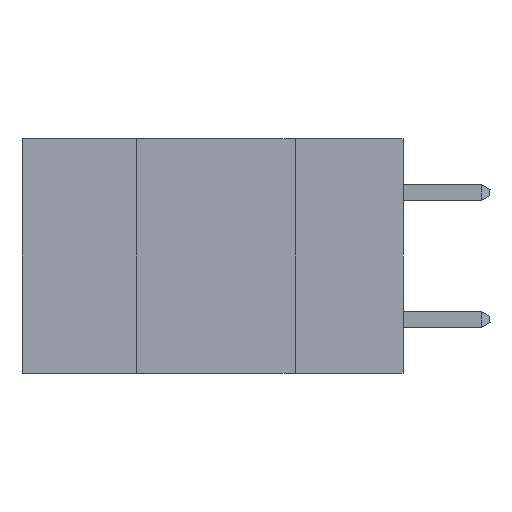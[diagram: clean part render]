
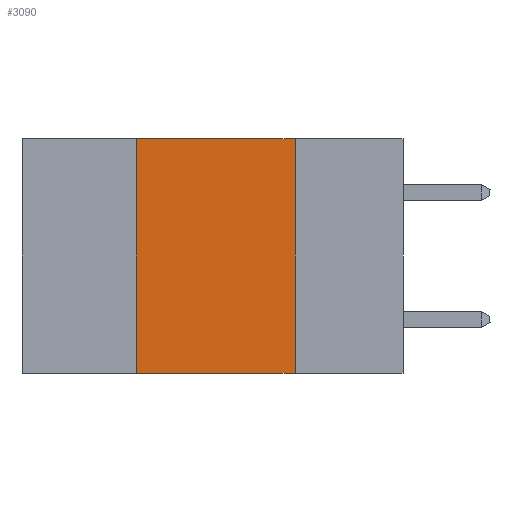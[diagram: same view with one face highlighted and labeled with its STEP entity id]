
A CAD part, left-side view. The second image highlights one B-rep face of the part: STEP entity #3090.
In plain terms, the highlighted planar face has unit normal (-1, 0, 0).
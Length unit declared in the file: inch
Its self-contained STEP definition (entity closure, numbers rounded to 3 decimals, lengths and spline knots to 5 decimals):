
#54 = EDGE_CURVE ( 'NONE', #2871, #9619, #1318, .T. ) ;
#426 = DIRECTION ( 'NONE',  ( 1., 0., 0. ) ) ;
#457 = AXIS2_PLACEMENT_3D ( 'NONE', #13632, #426, #7081 ) ;
#460 = CARTESIAN_POINT ( 'NONE',  ( 0., 0.42, 0. ) ) ;
#549 = EDGE_CURVE ( 'NONE', #13292, #9970, #6800, .T. ) ;
#629 = CARTESIAN_POINT ( 'NONE',  ( 0., 0.42, 0. ) ) ;
#1159 = VECTOR ( 'NONE', #8277, 39.37008 ) ;
#1318 = LINE ( 'NONE', #7548, #12963 ) ;
#2871 = VERTEX_POINT ( 'NONE', #11934 ) ;
#3051 = LINE ( 'NONE', #3916, #1159 ) ;
#3090 = ADVANCED_FACE ( 'NONE', ( #12786 ), #10303, .F. ) ;
#3916 = CARTESIAN_POINT ( 'NONE',  ( 0., 0.17, 0. ) ) ;
#4755 = CARTESIAN_POINT ( 'NONE',  ( 0., 0.17, -0.37 ) ) ;
#5334 = EDGE_CURVE ( 'NONE', #2871, #13292, #7919, .T. ) ;
#5450 = ORIENTED_EDGE ( 'NONE', *, *, #549, .F. ) ;
#5946 = DIRECTION ( 'NONE',  ( 0., 0., 1. ) ) ;
#6522 = CARTESIAN_POINT ( 'NONE',  ( 0., 0.17, 0. ) ) ;
#6800 = LINE ( 'NONE', #8638, #11696 ) ;
#7081 = DIRECTION ( 'NONE',  ( 0., 0., -1. ) ) ;
#7548 = CARTESIAN_POINT ( 'NONE',  ( 0., 0.6, -0.37 ) ) ;
#7919 = LINE ( 'NONE', #629, #8254 ) ;
#8254 = VECTOR ( 'NONE', #5946, 39.37008 ) ;
#8277 = DIRECTION ( 'NONE',  ( 0., 0., -1. ) ) ;
#8453 = DIRECTION ( 'NONE',  ( 0., -1., 0. ) ) ;
#8638 = CARTESIAN_POINT ( 'NONE',  ( 0., 0.6, 0. ) ) ;
#9619 = VERTEX_POINT ( 'NONE', #4755 ) ;
#9970 = VERTEX_POINT ( 'NONE', #6522 ) ;
#10150 = EDGE_LOOP ( 'NONE', ( #13589, #5450, #11818, #12194 ) ) ;
#10303 = PLANE ( 'NONE',  #457 ) ;
#10901 = DIRECTION ( 'NONE',  ( 0., -1., 0. ) ) ;
#11696 = VECTOR ( 'NONE', #8453, 39.37008 ) ;
#11818 = ORIENTED_EDGE ( 'NONE', *, *, #5334, .F. ) ;
#11934 = CARTESIAN_POINT ( 'NONE',  ( 0., 0.42, -0.37 ) ) ;
#12194 = ORIENTED_EDGE ( 'NONE', *, *, #54, .T. ) ;
#12786 = FACE_OUTER_BOUND ( 'NONE', #10150, .T. ) ;
#12963 = VECTOR ( 'NONE', #10901, 39.37008 ) ;
#13292 = VERTEX_POINT ( 'NONE', #460 ) ;
#13589 = ORIENTED_EDGE ( 'NONE', *, *, #14063, .F. ) ;
#13632 = CARTESIAN_POINT ( 'NONE',  ( 0., 0.6, 0. ) ) ;
#14063 = EDGE_CURVE ( 'NONE', #9970, #9619, #3051, .T. ) ;
